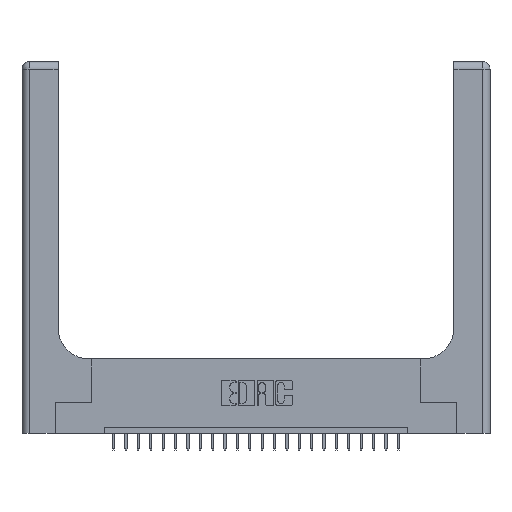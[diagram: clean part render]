
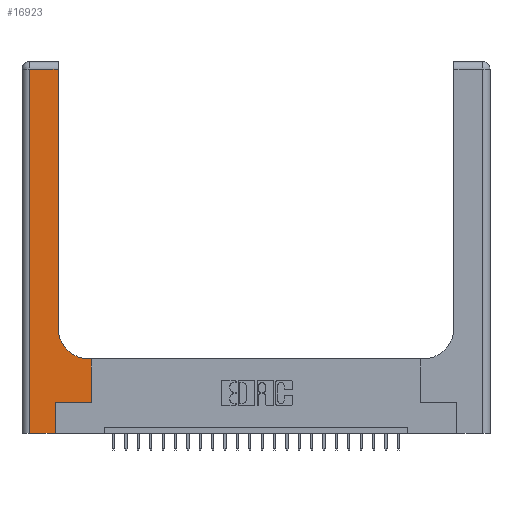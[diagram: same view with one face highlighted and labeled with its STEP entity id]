
A CAD part, top view. The second image highlights one B-rep face of the part: STEP entity #16923.
In plain terms, the highlighted planar face has unit normal (0, 0, 1).
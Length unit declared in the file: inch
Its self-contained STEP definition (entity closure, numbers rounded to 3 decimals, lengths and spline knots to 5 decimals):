
#16 = LINE ( 'NONE', #4181, #12217 ) ;
#235 = CARTESIAN_POINT ( 'NONE',  ( 0., 2.94, 0.37 ) ) ;
#593 = DIRECTION ( 'NONE',  ( 1., 0., 0. ) ) ;
#915 = VECTOR ( 'NONE', #8414, 39.37008 ) ;
#1575 = LINE ( 'NONE', #5431, #14703 ) ;
#2044 = FACE_OUTER_BOUND ( 'NONE', #9821, .T. ) ;
#2221 = DIRECTION ( 'NONE',  ( 0., 1., 0. ) ) ;
#3180 = DIRECTION ( 'NONE',  ( 0., 0., -1. ) ) ;
#3459 = DIRECTION ( 'NONE',  ( -1., 0., 0. ) ) ;
#3638 = CARTESIAN_POINT ( 'NONE',  ( 0.269, 0., 0.37 ) ) ;
#3705 = EDGE_CURVE ( 'NONE', #8387, #22076, #1575, .T. ) ;
#3790 = DIRECTION ( 'NONE',  ( 1., 0., 0. ) ) ;
#3832 = LINE ( 'NONE', #13473, #15367 ) ;
#4008 = LINE ( 'NONE', #5730, #6890 ) ;
#4181 = CARTESIAN_POINT ( 'NONE',  ( 0.5585, 0.25, 0.37 ) ) ;
#4268 = CARTESIAN_POINT ( 'NONE',  ( 0.2915, 3., 0.37 ) ) ;
#4321 = EDGE_CURVE ( 'NONE', #22076, #21633, #13933, .T. ) ;
#4634 = CARTESIAN_POINT ( 'NONE',  ( 0.269, 0.25, 0.37 ) ) ;
#5431 = CARTESIAN_POINT ( 'NONE',  ( 0.2915, 0.6, 0.37 ) ) ;
#5573 = EDGE_CURVE ( 'NONE', #9349, #22375, #10761, .T. ) ;
#5730 = CARTESIAN_POINT ( 'NONE',  ( 0.269, 0., 0.37 ) ) ;
#5897 = ORIENTED_EDGE ( 'NONE', *, *, #23750, .T. ) ;
#5949 = EDGE_CURVE ( 'NONE', #18713, #6140, #3832, .T. ) ;
#6140 = VERTEX_POINT ( 'NONE', #6559 ) ;
#6264 = CARTESIAN_POINT ( 'NONE',  ( 0., 0., 0.37 ) ) ;
#6531 = CARTESIAN_POINT ( 'NONE',  ( 0.5415, 0.6, 0.37 ) ) ;
#6559 = CARTESIAN_POINT ( 'NONE',  ( 0.06, 0., 0.37 ) ) ;
#6890 = VECTOR ( 'NONE', #15838, 39.37008 ) ;
#7390 = ORIENTED_EDGE ( 'NONE', *, *, #3705, .T. ) ;
#7480 = DIRECTION ( 'NONE',  ( 0., -1., 0. ) ) ;
#8296 = EDGE_CURVE ( 'NONE', #6140, #12429, #24118, .T. ) ;
#8387 = VERTEX_POINT ( 'NONE', #22542 ) ;
#8414 = DIRECTION ( 'NONE',  ( -1., 0., 0. ) ) ;
#8545 = CARTESIAN_POINT ( 'NONE',  ( 0.269, 0.25, 0.37 ) ) ;
#9285 = EDGE_CURVE ( 'NONE', #14048, #18713, #12212, .T. ) ;
#9349 = VERTEX_POINT ( 'NONE', #8545 ) ;
#9821 = EDGE_LOOP ( 'NONE', ( #5897, #18290, #25636, #23901, #16560, #20312, #14764, #7390, #18203 ) ) ;
#10369 = LINE ( 'NONE', #4268, #12182 ) ;
#10495 = DIRECTION ( 'NONE',  ( 0., 1., 0. ) ) ;
#10578 = DIRECTION ( 'NONE',  ( 0., 0., -1. ) ) ;
#10760 = PLANE ( 'NONE',  #17326 ) ;
#10761 = LINE ( 'NONE', #4634, #24229 ) ;
#10861 = EDGE_CURVE ( 'NONE', #22375, #8387, #16, .T. ) ;
#10914 = CARTESIAN_POINT ( 'NONE',  ( 0.5585, 0.25, 0.37 ) ) ;
#11028 = AXIS2_PLACEMENT_3D ( 'NONE', #22829, #10578, #20462 ) ;
#12182 = VECTOR ( 'NONE', #10495, 39.37008 ) ;
#12212 = LINE ( 'NONE', #235, #915 ) ;
#12217 = VECTOR ( 'NONE', #2221, 39.37008 ) ;
#12429 = VERTEX_POINT ( 'NONE', #3638 ) ;
#13377 = EDGE_CURVE ( 'NONE', #12429, #9349, #4008, .T. ) ;
#13473 = CARTESIAN_POINT ( 'NONE',  ( 0.06, 3., 0.37 ) ) ;
#13933 = CIRCLE ( 'NONE', #11028, 0.25 ) ;
#14048 = VERTEX_POINT ( 'NONE', #15066 ) ;
#14703 = VECTOR ( 'NONE', #3459, 39.37008 ) ;
#14764 = ORIENTED_EDGE ( 'NONE', *, *, #10861, .T. ) ;
#15066 = CARTESIAN_POINT ( 'NONE',  ( 0.2915, 2.94, 0.37 ) ) ;
#15367 = VECTOR ( 'NONE', #7480, 39.37008 ) ;
#15838 = DIRECTION ( 'NONE',  ( 0., 1., 0. ) ) ;
#16560 = ORIENTED_EDGE ( 'NONE', *, *, #13377, .T. ) ;
#16923 = ADVANCED_FACE ( 'NONE', ( #2044 ), #10760, .F. ) ;
#17326 = AXIS2_PLACEMENT_3D ( 'NONE', #22993, #3180, #19038 ) ;
#17403 = CARTESIAN_POINT ( 'NONE',  ( 0.2915, 0.85, 0.37 ) ) ;
#18203 = ORIENTED_EDGE ( 'NONE', *, *, #4321, .T. ) ;
#18290 = ORIENTED_EDGE ( 'NONE', *, *, #9285, .T. ) ;
#18713 = VERTEX_POINT ( 'NONE', #24614 ) ;
#19038 = DIRECTION ( 'NONE',  ( -1., 0., 0. ) ) ;
#20312 = ORIENTED_EDGE ( 'NONE', *, *, #5573, .T. ) ;
#20462 = DIRECTION ( 'NONE',  ( 1., 0., 0. ) ) ;
#21633 = VERTEX_POINT ( 'NONE', #17403 ) ;
#22076 = VERTEX_POINT ( 'NONE', #6531 ) ;
#22375 = VERTEX_POINT ( 'NONE', #10914 ) ;
#22542 = CARTESIAN_POINT ( 'NONE',  ( 0.5585, 0.6, 0.37 ) ) ;
#22829 = CARTESIAN_POINT ( 'NONE',  ( 0.5415, 0.85, 0.37 ) ) ;
#22993 = CARTESIAN_POINT ( 'NONE',  ( 0., 3., 0.37 ) ) ;
#23004 = VECTOR ( 'NONE', #3790, 39.37008 ) ;
#23750 = EDGE_CURVE ( 'NONE', #21633, #14048, #10369, .T. ) ;
#23901 = ORIENTED_EDGE ( 'NONE', *, *, #8296, .T. ) ;
#24118 = LINE ( 'NONE', #6264, #23004 ) ;
#24229 = VECTOR ( 'NONE', #593, 39.37008 ) ;
#24614 = CARTESIAN_POINT ( 'NONE',  ( 0.06, 2.94, 0.37 ) ) ;
#25636 = ORIENTED_EDGE ( 'NONE', *, *, #5949, .T. ) ;
